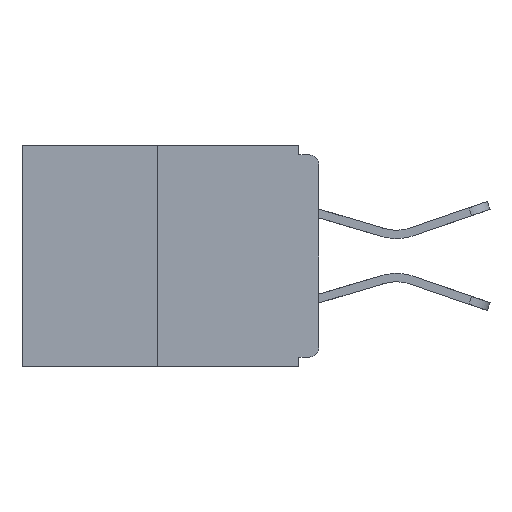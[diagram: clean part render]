
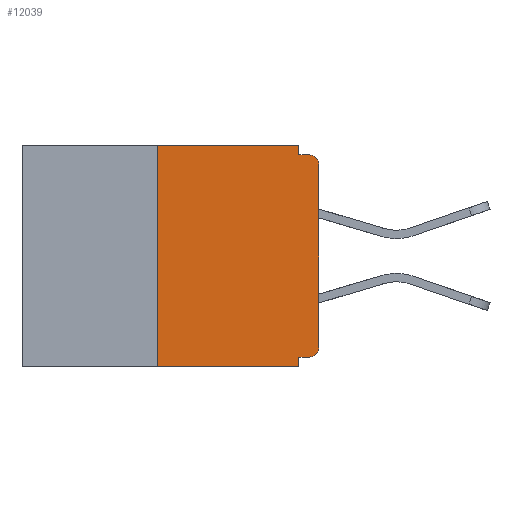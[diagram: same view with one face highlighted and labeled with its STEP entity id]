
A CAD part, left-side view. The second image highlights one B-rep face of the part: STEP entity #12039.
In plain terms, the highlighted planar face has unit normal (-1, 0, 0).
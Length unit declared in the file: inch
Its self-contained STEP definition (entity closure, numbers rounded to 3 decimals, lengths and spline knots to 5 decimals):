
#59 = DIRECTION ( 'NONE',  ( 0., 0., 1. ) ) ;
#110 = CARTESIAN_POINT ( 'NONE',  ( 0., 0., -0.313 ) ) ;
#406 = LINE ( 'NONE', #11842, #9993 ) ;
#950 = VERTEX_POINT ( 'NONE', #15076 ) ;
#1081 = CARTESIAN_POINT ( 'NONE',  ( 0., 0.031, -0.343 ) ) ;
#1241 = CARTESIAN_POINT ( 'NONE',  ( 0., 0.031, 0. ) ) ;
#1332 = DIRECTION ( 'NONE',  ( 0., 1., 0. ) ) ;
#1357 = EDGE_CURVE ( 'NONE', #11327, #8734, #1474, .T. ) ;
#1474 = CIRCLE ( 'NONE', #6047, 0.015 ) ;
#1650 = DIRECTION ( 'NONE',  ( 1., 0., 0. ) ) ;
#2078 = VECTOR ( 'NONE', #4258, 39.37008 ) ;
#2129 = EDGE_CURVE ( 'NONE', #14712, #10956, #14449, .T. ) ;
#2388 = AXIS2_PLACEMENT_3D ( 'NONE', #14888, #1650, #11288 ) ;
#2416 = ORIENTED_EDGE ( 'NONE', *, *, #5234, .F. ) ;
#2508 = CARTESIAN_POINT ( 'NONE',  ( 0., 0., -0.328 ) ) ;
#2571 = ORIENTED_EDGE ( 'NONE', *, *, #6605, .F. ) ;
#2603 = CARTESIAN_POINT ( 'NONE',  ( 0., 0.25, 0. ) ) ;
#2662 = ORIENTED_EDGE ( 'NONE', *, *, #2129, .F. ) ;
#2770 = CARTESIAN_POINT ( 'NONE',  ( 0., 0.031, -0.343 ) ) ;
#3177 = DIRECTION ( 'NONE',  ( 0., 0., -1. ) ) ;
#3416 = CARTESIAN_POINT ( 'NONE',  ( 0., 0.25, 0. ) ) ;
#3626 = LINE ( 'NONE', #13794, #12484 ) ;
#4179 = EDGE_CURVE ( 'NONE', #950, #13852, #5711, .T. ) ;
#4258 = DIRECTION ( 'NONE',  ( 0., -1., 0. ) ) ;
#4347 = EDGE_CURVE ( 'NONE', #13852, #11327, #3626, .T. ) ;
#4578 = EDGE_LOOP ( 'NONE', ( #2416, #2571, #4933, #5807, #12826, #10821, #6068, #8514, #15009, #2662 ) ) ;
#4660 = DIRECTION ( 'NONE',  ( 0., -1., 0. ) ) ;
#4708 = DIRECTION ( 'NONE',  ( 0., 0., -1. ) ) ;
#4933 = ORIENTED_EDGE ( 'NONE', *, *, #5122, .T. ) ;
#4989 = LINE ( 'NONE', #3416, #13068 ) ;
#5122 = EDGE_CURVE ( 'NONE', #13306, #11011, #9649, .T. ) ;
#5188 = PLANE ( 'NONE',  #2388 ) ;
#5234 = EDGE_CURVE ( 'NONE', #9051, #14712, #14554, .T. ) ;
#5711 = CIRCLE ( 'NONE', #9718, 0.015 ) ;
#5807 = ORIENTED_EDGE ( 'NONE', *, *, #9540, .F. ) ;
#6047 = AXIS2_PLACEMENT_3D ( 'NONE', #8469, #7096, #8351 ) ;
#6068 = ORIENTED_EDGE ( 'NONE', *, *, #4347, .T. ) ;
#6337 = CARTESIAN_POINT ( 'NONE',  ( 0., 0.015, -0.313 ) ) ;
#6605 = EDGE_CURVE ( 'NONE', #13306, #9051, #4989, .T. ) ;
#7096 = DIRECTION ( 'NONE',  ( -1., 0., 0. ) ) ;
#7707 = CARTESIAN_POINT ( 'NONE',  ( 0., 0.031, 0. ) ) ;
#7765 = CARTESIAN_POINT ( 'NONE',  ( 0., 0.46, -0.343 ) ) ;
#7767 = VERTEX_POINT ( 'NONE', #10681 ) ;
#7864 = DIRECTION ( 'NONE',  ( -1., 0., 0. ) ) ;
#8150 = VECTOR ( 'NONE', #13223, 39.37008 ) ;
#8351 = DIRECTION ( 'NONE',  ( 0., 0., -1. ) ) ;
#8469 = CARTESIAN_POINT ( 'NONE',  ( 0., 0.015, -0.03 ) ) ;
#8502 = DIRECTION ( 'NONE',  ( 0., 0., -1. ) ) ;
#8514 = ORIENTED_EDGE ( 'NONE', *, *, #1357, .T. ) ;
#8585 = CARTESIAN_POINT ( 'NONE',  ( 0., 0.031, -0.015 ) ) ;
#8734 = VERTEX_POINT ( 'NONE', #12672 ) ;
#8812 = VECTOR ( 'NONE', #8502, 39.37008 ) ;
#9051 = VERTEX_POINT ( 'NONE', #2603 ) ;
#9540 = EDGE_CURVE ( 'NONE', #7767, #11011, #14298, .T. ) ;
#9649 = LINE ( 'NONE', #7765, #2078 ) ;
#9718 = AXIS2_PLACEMENT_3D ( 'NONE', #6337, #7864, #3177 ) ;
#9860 = FACE_OUTER_BOUND ( 'NONE', #4578, .T. ) ;
#9895 = CARTESIAN_POINT ( 'NONE',  ( 0., 0.25, -0.343 ) ) ;
#9993 = VECTOR ( 'NONE', #4660, 39.37008 ) ;
#10010 = DIRECTION ( 'NONE',  ( 0., 0., 1. ) ) ;
#10336 = VECTOR ( 'NONE', #4708, 39.37008 ) ;
#10681 = CARTESIAN_POINT ( 'NONE',  ( 0., 0.031, -0.328 ) ) ;
#10790 = CARTESIAN_POINT ( 'NONE',  ( 0., 0., -0.03 ) ) ;
#10821 = ORIENTED_EDGE ( 'NONE', *, *, #4179, .T. ) ;
#10956 = VERTEX_POINT ( 'NONE', #8585 ) ;
#11011 = VERTEX_POINT ( 'NONE', #2770 ) ;
#11288 = DIRECTION ( 'NONE',  ( 0., 0., -1. ) ) ;
#11327 = VERTEX_POINT ( 'NONE', #10790 ) ;
#11392 = EDGE_CURVE ( 'NONE', #950, #7767, #14465, .T. ) ;
#11607 = VECTOR ( 'NONE', #1332, 39.37008 ) ;
#11842 = CARTESIAN_POINT ( 'NONE',  ( 0., 0., -0.015 ) ) ;
#12039 = ADVANCED_FACE ( 'NONE', ( #9860 ), #5188, .F. ) ;
#12222 = CARTESIAN_POINT ( 'NONE',  ( 0., 0.46, 0. ) ) ;
#12484 = VECTOR ( 'NONE', #10010, 39.37008 ) ;
#12672 = CARTESIAN_POINT ( 'NONE',  ( 0., 0.015, -0.015 ) ) ;
#12826 = ORIENTED_EDGE ( 'NONE', *, *, #11392, .F. ) ;
#13068 = VECTOR ( 'NONE', #59, 39.37008 ) ;
#13223 = DIRECTION ( 'NONE',  ( 0., -1., 0. ) ) ;
#13306 = VERTEX_POINT ( 'NONE', #9895 ) ;
#13672 = EDGE_CURVE ( 'NONE', #10956, #8734, #406, .T. ) ;
#13794 = CARTESIAN_POINT ( 'NONE',  ( 0., 0., 0. ) ) ;
#13852 = VERTEX_POINT ( 'NONE', #110 ) ;
#14298 = LINE ( 'NONE', #1081, #10336 ) ;
#14449 = LINE ( 'NONE', #1241, #8812 ) ;
#14465 = LINE ( 'NONE', #2508, #11607 ) ;
#14554 = LINE ( 'NONE', #12222, #8150 ) ;
#14712 = VERTEX_POINT ( 'NONE', #7707 ) ;
#14888 = CARTESIAN_POINT ( 'NONE',  ( 0., 0.46, 0. ) ) ;
#15009 = ORIENTED_EDGE ( 'NONE', *, *, #13672, .F. ) ;
#15076 = CARTESIAN_POINT ( 'NONE',  ( 0., 0.015, -0.328 ) ) ;
